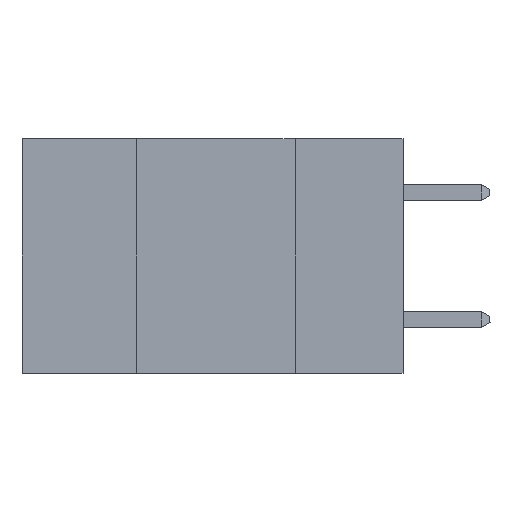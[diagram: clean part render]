
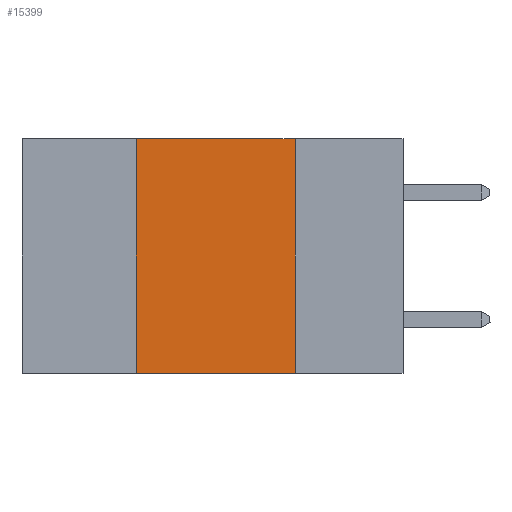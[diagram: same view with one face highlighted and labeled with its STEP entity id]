
A CAD part, left-side view. The second image highlights one B-rep face of the part: STEP entity #15399.
In plain terms, the highlighted planar face has unit normal (-1, 0, 0).
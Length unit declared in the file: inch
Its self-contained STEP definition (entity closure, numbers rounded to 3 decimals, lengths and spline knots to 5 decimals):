
#205 = CARTESIAN_POINT ( 'NONE',  ( 0., 0.6, 0. ) ) ;
#797 = FACE_OUTER_BOUND ( 'NONE', #12167, .T. ) ;
#1754 = DIRECTION ( 'NONE',  ( 0., 0., -1. ) ) ;
#1965 = DIRECTION ( 'NONE',  ( 1., 0., 0. ) ) ;
#2018 = CARTESIAN_POINT ( 'NONE',  ( 0., 0.17, -0.37 ) ) ;
#3293 = ORIENTED_EDGE ( 'NONE', *, *, #11110, .F. ) ;
#3340 = CARTESIAN_POINT ( 'NONE',  ( 0., 0.42, -0.37 ) ) ;
#3550 = ORIENTED_EDGE ( 'NONE', *, *, #17019, .T. ) ;
#3587 = ORIENTED_EDGE ( 'NONE', *, *, #7463, .F. ) ;
#5287 = CARTESIAN_POINT ( 'NONE',  ( 0., 0.17, 0. ) ) ;
#5781 = VERTEX_POINT ( 'NONE', #3340 ) ;
#5814 = CARTESIAN_POINT ( 'NONE',  ( 0., 0.6, -0.37 ) ) ;
#6115 = AXIS2_PLACEMENT_3D ( 'NONE', #205, #1965, #13764 ) ;
#6257 = VECTOR ( 'NONE', #16867, 39.37008 ) ;
#6574 = VERTEX_POINT ( 'NONE', #5287 ) ;
#7315 = LINE ( 'NONE', #15102, #6257 ) ;
#7463 = EDGE_CURVE ( 'NONE', #5781, #13278, #19056, .T. ) ;
#8043 = CARTESIAN_POINT ( 'NONE',  ( 0., 0.42, 0. ) ) ;
#8363 = CARTESIAN_POINT ( 'NONE',  ( 0., 0.17, 0. ) ) ;
#8981 = ORIENTED_EDGE ( 'NONE', *, *, #13116, .F. ) ;
#9334 = VECTOR ( 'NONE', #1754, 39.37008 ) ;
#9437 = VECTOR ( 'NONE', #17736, 39.37008 ) ;
#9859 = LINE ( 'NONE', #8363, #9334 ) ;
#10339 = PLANE ( 'NONE',  #6115 ) ;
#11110 = EDGE_CURVE ( 'NONE', #13278, #6574, #7315, .T. ) ;
#12167 = EDGE_LOOP ( 'NONE', ( #8981, #3293, #3587, #3550 ) ) ;
#13116 = EDGE_CURVE ( 'NONE', #6574, #16135, #9859, .T. ) ;
#13278 = VERTEX_POINT ( 'NONE', #19127 ) ;
#13764 = DIRECTION ( 'NONE',  ( 0., 0., -1. ) ) ;
#13919 = VECTOR ( 'NONE', #21699, 39.37008 ) ;
#13930 = LINE ( 'NONE', #5814, #9437 ) ;
#15102 = CARTESIAN_POINT ( 'NONE',  ( 0., 0.6, 0. ) ) ;
#15399 = ADVANCED_FACE ( 'NONE', ( #797 ), #10339, .F. ) ;
#16135 = VERTEX_POINT ( 'NONE', #2018 ) ;
#16867 = DIRECTION ( 'NONE',  ( 0., -1., 0. ) ) ;
#17019 = EDGE_CURVE ( 'NONE', #5781, #16135, #13930, .T. ) ;
#17736 = DIRECTION ( 'NONE',  ( 0., -1., 0. ) ) ;
#19056 = LINE ( 'NONE', #8043, #13919 ) ;
#19127 = CARTESIAN_POINT ( 'NONE',  ( 0., 0.42, 0. ) ) ;
#21699 = DIRECTION ( 'NONE',  ( 0., 0., 1. ) ) ;
